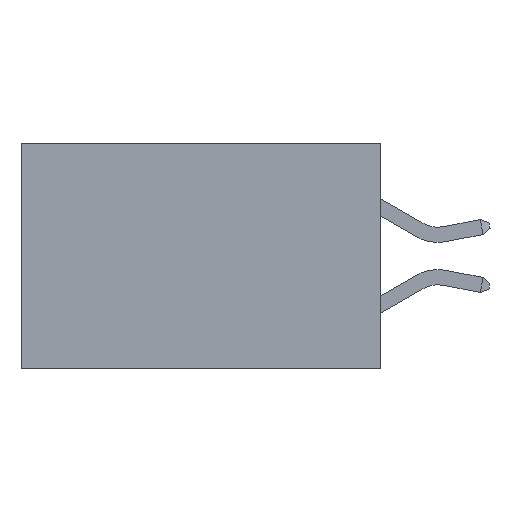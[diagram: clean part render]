
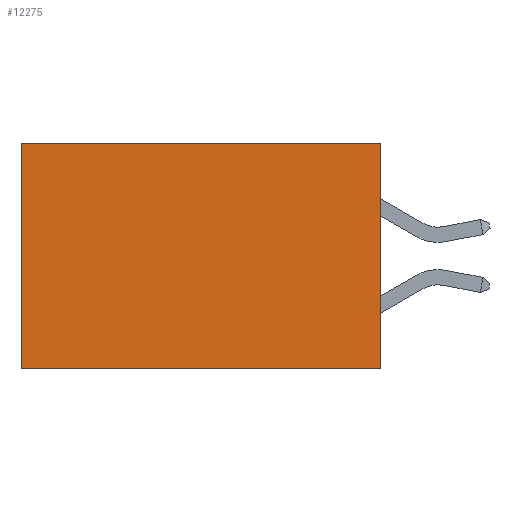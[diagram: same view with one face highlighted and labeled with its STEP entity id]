
A CAD part, left-side view. The second image highlights one B-rep face of the part: STEP entity #12275.
In plain terms, the highlighted planar face has unit normal (-1, 0, 0).
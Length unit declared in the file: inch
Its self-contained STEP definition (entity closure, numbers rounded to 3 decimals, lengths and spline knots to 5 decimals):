
#65 = FACE_OUTER_BOUND ( 'NONE', #8421, .T. ) ;
#1462 = VECTOR ( 'NONE', #15193, 39.37008 ) ;
#1617 = VERTEX_POINT ( 'NONE', #16777 ) ;
#1994 = DIRECTION ( 'NONE',  ( 0., 0., -1. ) ) ;
#2856 = ORIENTED_EDGE ( 'NONE', *, *, #22063, .T. ) ;
#3818 = CARTESIAN_POINT ( 'NONE',  ( 0.277, 0.59, 0. ) ) ;
#6402 = LINE ( 'NONE', #13308, #1462 ) ;
#6723 = CARTESIAN_POINT ( 'NONE',  ( 0.277, 0., -0.37 ) ) ;
#8143 = EDGE_CURVE ( 'NONE', #9933, #12678, #9879, .T. ) ;
#8420 = LINE ( 'NONE', #11400, #22792 ) ;
#8421 = EDGE_LOOP ( 'NONE', ( #14552, #14335, #10904, #2856 ) ) ;
#9581 = DIRECTION ( 'NONE',  ( 0., 1., 0. ) ) ;
#9879 = LINE ( 'NONE', #15823, #14268 ) ;
#9933 = VERTEX_POINT ( 'NONE', #16691 ) ;
#10904 = ORIENTED_EDGE ( 'NONE', *, *, #8143, .F. ) ;
#11300 = CARTESIAN_POINT ( 'NONE',  ( 0.277, 0., 0. ) ) ;
#11400 = CARTESIAN_POINT ( 'NONE',  ( 0.277, 0., -0.37 ) ) ;
#11465 = PLANE ( 'NONE',  #18959 ) ;
#12275 = ADVANCED_FACE ( 'NONE', ( #65 ), #11465, .F. ) ;
#12678 = VERTEX_POINT ( 'NONE', #6723 ) ;
#12780 = LINE ( 'NONE', #11300, #22666 ) ;
#13308 = CARTESIAN_POINT ( 'NONE',  ( 0.277, 0.59, -0.37 ) ) ;
#13350 = DIRECTION ( 'NONE',  ( 1., 0., 0. ) ) ;
#14268 = VECTOR ( 'NONE', #14645, 39.37008 ) ;
#14335 = ORIENTED_EDGE ( 'NONE', *, *, #18303, .F. ) ;
#14552 = ORIENTED_EDGE ( 'NONE', *, *, #16367, .T. ) ;
#14645 = DIRECTION ( 'NONE',  ( 0., 0., -1. ) ) ;
#15193 = DIRECTION ( 'NONE',  ( 0., 0., -1. ) ) ;
#15823 = CARTESIAN_POINT ( 'NONE',  ( 0.277, 0., -0.37 ) ) ;
#16367 = EDGE_CURVE ( 'NONE', #23469, #1617, #6402, .T. ) ;
#16691 = CARTESIAN_POINT ( 'NONE',  ( 0.277, 0., 0. ) ) ;
#16777 = CARTESIAN_POINT ( 'NONE',  ( 0.277, 0.59, -0.37 ) ) ;
#16996 = CARTESIAN_POINT ( 'NONE',  ( 0.277, 0., -0.37 ) ) ;
#18303 = EDGE_CURVE ( 'NONE', #12678, #1617, #8420, .T. ) ;
#18959 = AXIS2_PLACEMENT_3D ( 'NONE', #16996, #13350, #1994 ) ;
#22063 = EDGE_CURVE ( 'NONE', #9933, #23469, #12780, .T. ) ;
#22450 = DIRECTION ( 'NONE',  ( 0., 1., 0. ) ) ;
#22666 = VECTOR ( 'NONE', #22450, 39.37008 ) ;
#22792 = VECTOR ( 'NONE', #9581, 39.37008 ) ;
#23469 = VERTEX_POINT ( 'NONE', #3818 ) ;
